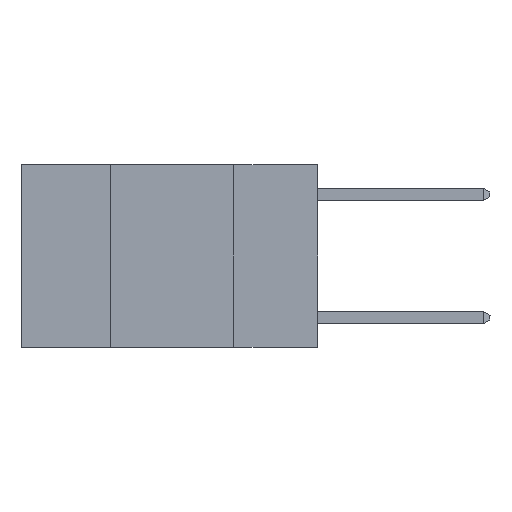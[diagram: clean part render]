
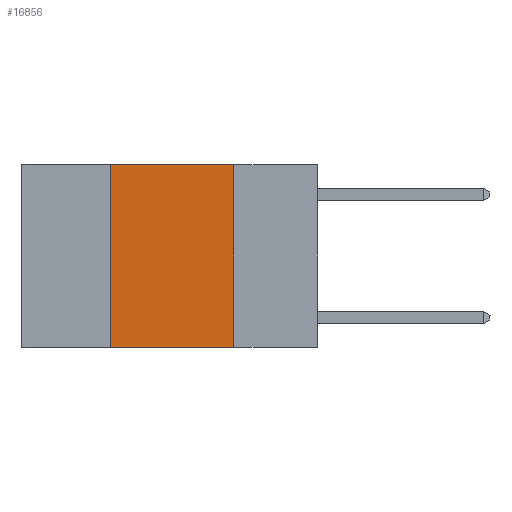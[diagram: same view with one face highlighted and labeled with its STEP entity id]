
A CAD part, left-side view. The second image highlights one B-rep face of the part: STEP entity #16856.
In plain terms, the highlighted planar face has unit normal (-1, 0, 0).
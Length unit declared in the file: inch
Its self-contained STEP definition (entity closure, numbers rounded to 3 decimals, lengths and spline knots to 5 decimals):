
#236 = CARTESIAN_POINT ( 'NONE',  ( 0., 0.17, -0.37 ) ) ;
#505 = DIRECTION ( 'NONE',  ( 0., 0., 1. ) ) ;
#1918 = VERTEX_POINT ( 'NONE', #236 ) ;
#2085 = VERTEX_POINT ( 'NONE', #9949 ) ;
#2575 = DIRECTION ( 'NONE',  ( 0., -1., 0. ) ) ;
#2821 = EDGE_LOOP ( 'NONE', ( #11511, #13764, #15817, #13292 ) ) ;
#3340 = CARTESIAN_POINT ( 'NONE',  ( 0., 0.6, 0. ) ) ;
#3686 = EDGE_CURVE ( 'NONE', #12098, #1918, #14109, .T. ) ;
#4088 = LINE ( 'NONE', #9822, #19812 ) ;
#5623 = PLANE ( 'NONE',  #19505 ) ;
#5847 = VERTEX_POINT ( 'NONE', #13297 ) ;
#6573 = LINE ( 'NONE', #10352, #17828 ) ;
#7191 = DIRECTION ( 'NONE',  ( 0., 0., -1. ) ) ;
#8709 = CARTESIAN_POINT ( 'NONE',  ( 0., 0.6, 0. ) ) ;
#8767 = DIRECTION ( 'NONE',  ( 0., 0., -1. ) ) ;
#9822 = CARTESIAN_POINT ( 'NONE',  ( 0., 0.42, 0. ) ) ;
#9949 = CARTESIAN_POINT ( 'NONE',  ( 0., 0.42, 0. ) ) ;
#10016 = EDGE_CURVE ( 'NONE', #5847, #2085, #4088, .T. ) ;
#10352 = CARTESIAN_POINT ( 'NONE',  ( 0., 0.6, -0.37 ) ) ;
#11316 = VECTOR ( 'NONE', #17174, 39.37008 ) ;
#11376 = FACE_OUTER_BOUND ( 'NONE', #2821, .T. ) ;
#11511 = ORIENTED_EDGE ( 'NONE', *, *, #3686, .F. ) ;
#11875 = CARTESIAN_POINT ( 'NONE',  ( 0., 0.17, 0. ) ) ;
#12098 = VERTEX_POINT ( 'NONE', #14598 ) ;
#12540 = EDGE_CURVE ( 'NONE', #2085, #12098, #15297, .T. ) ;
#13292 = ORIENTED_EDGE ( 'NONE', *, *, #19418, .T. ) ;
#13297 = CARTESIAN_POINT ( 'NONE',  ( 0., 0.42, -0.37 ) ) ;
#13650 = VECTOR ( 'NONE', #8767, 39.37008 ) ;
#13764 = ORIENTED_EDGE ( 'NONE', *, *, #12540, .F. ) ;
#14109 = LINE ( 'NONE', #11875, #13650 ) ;
#14598 = CARTESIAN_POINT ( 'NONE',  ( 0., 0.17, 0. ) ) ;
#15297 = LINE ( 'NONE', #3340, #11316 ) ;
#15817 = ORIENTED_EDGE ( 'NONE', *, *, #10016, .F. ) ;
#16353 = DIRECTION ( 'NONE',  ( 1., 0., 0. ) ) ;
#16856 = ADVANCED_FACE ( 'NONE', ( #11376 ), #5623, .F. ) ;
#17174 = DIRECTION ( 'NONE',  ( 0., -1., 0. ) ) ;
#17828 = VECTOR ( 'NONE', #2575, 39.37008 ) ;
#19418 = EDGE_CURVE ( 'NONE', #5847, #1918, #6573, .T. ) ;
#19505 = AXIS2_PLACEMENT_3D ( 'NONE', #8709, #16353, #7191 ) ;
#19812 = VECTOR ( 'NONE', #505, 39.37008 ) ;
